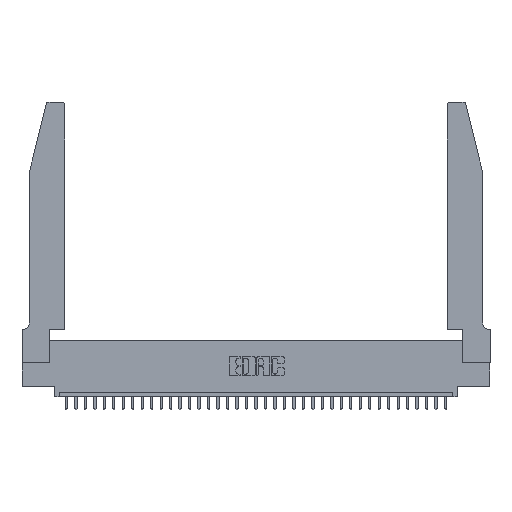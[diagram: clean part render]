
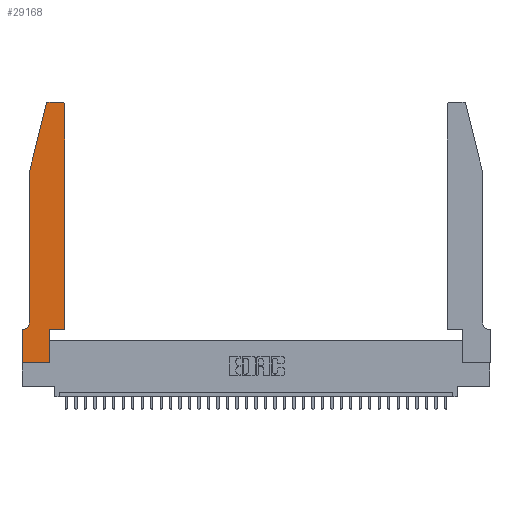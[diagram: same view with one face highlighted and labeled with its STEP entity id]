
A CAD part, top view. The second image highlights one B-rep face of the part: STEP entity #29168.
In plain terms, the highlighted planar face has unit normal (0, 0, 1).
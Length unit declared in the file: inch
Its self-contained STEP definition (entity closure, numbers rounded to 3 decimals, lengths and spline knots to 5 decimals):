
#241 = CARTESIAN_POINT ( 'NONE',  ( 0.0755, 0.42, 0.37 ) ) ;
#341 = EDGE_CURVE ( 'NONE', #12670, #24252, #7398, .T. ) ;
#362 = EDGE_CURVE ( 'NONE', #797, #8042, #8285, .T. ) ;
#366 = DIRECTION ( 'NONE',  ( 0., -1., 0. ) ) ;
#797 = VERTEX_POINT ( 'NONE', #11339 ) ;
#2567 = CARTESIAN_POINT ( 'NONE',  ( 0.2865, 0.35, 0.37 ) ) ;
#3261 = VERTEX_POINT ( 'NONE', #241 ) ;
#4064 = VECTOR ( 'NONE', #11460, 39.37008 ) ;
#4158 = CARTESIAN_POINT ( 'NONE',  ( 0.4505, 0.35, 0.37 ) ) ;
#4185 = ORIENTED_EDGE ( 'NONE', *, *, #7648, .T. ) ;
#4547 = DIRECTION ( 'NONE',  ( -1., 0., 0. ) ) ;
#5834 = LINE ( 'NONE', #22828, #4064 ) ;
#6407 = DIRECTION ( 'NONE',  ( -1., 0., 0. ) ) ;
#6819 = CARTESIAN_POINT ( 'NONE',  ( 0.0755, 2., 0.37 ) ) ;
#6827 = FACE_OUTER_BOUND ( 'NONE', #21174, .T. ) ;
#6879 = DIRECTION ( 'NONE',  ( 1., 0., 0. ) ) ;
#7135 = CARTESIAN_POINT ( 'NONE',  ( 0.4205, 2.72, 0.37 ) ) ;
#7398 = LINE ( 'NONE', #17165, #31655 ) ;
#7491 = DIRECTION ( 'NONE',  ( 0., 0., -1. ) ) ;
#7648 = EDGE_CURVE ( 'NONE', #17571, #33797, #11911, .T. ) ;
#7782 = AXIS2_PLACEMENT_3D ( 'NONE', #21209, #7491, #4547 ) ;
#8014 = VERTEX_POINT ( 'NONE', #6819 ) ;
#8042 = VERTEX_POINT ( 'NONE', #15754 ) ;
#8096 = CARTESIAN_POINT ( 'NONE',  ( 0.0055, 0.35, 0.37 ) ) ;
#8285 = LINE ( 'NONE', #28134, #21728 ) ;
#8612 = DIRECTION ( 'NONE',  ( -0.239, -0.971, 0. ) ) ;
#9207 = LINE ( 'NONE', #25236, #26567 ) ;
#9982 = EDGE_CURVE ( 'NONE', #12471, #8014, #9207, .T. ) ;
#10126 = DIRECTION ( 'NONE',  ( 1., 0., 0. ) ) ;
#10306 = EDGE_CURVE ( 'NONE', #33797, #12670, #18349, .T. ) ;
#10959 = LINE ( 'NONE', #15332, #23095 ) ;
#11264 = ORIENTED_EDGE ( 'NONE', *, *, #26913, .T. ) ;
#11339 = CARTESIAN_POINT ( 'NONE',  ( 0.4205, 2.75, 0.37 ) ) ;
#11460 = DIRECTION ( 'NONE',  ( 1., 0., 0. ) ) ;
#11486 = ORIENTED_EDGE ( 'NONE', *, *, #341, .T. ) ;
#11681 = DIRECTION ( 'NONE',  ( -1., 0., 0. ) ) ;
#11911 = LINE ( 'NONE', #14180, #27510 ) ;
#12445 = VERTEX_POINT ( 'NONE', #26707 ) ;
#12471 = VERTEX_POINT ( 'NONE', #34556 ) ;
#12670 = VERTEX_POINT ( 'NONE', #33101 ) ;
#13048 = EDGE_CURVE ( 'NONE', #12445, #797, #20366, .T. ) ;
#13626 = DIRECTION ( 'NONE',  ( 1., 0., 0. ) ) ;
#14049 = AXIS2_PLACEMENT_3D ( 'NONE', #24625, #27410, #13626 ) ;
#14180 = CARTESIAN_POINT ( 'NONE',  ( 0., 0., 0.37 ) ) ;
#15332 = CARTESIAN_POINT ( 'NONE',  ( 0.0755, 0.35, 0.37 ) ) ;
#15754 = CARTESIAN_POINT ( 'NONE',  ( 0.284, 2.75, 0.37 ) ) ;
#16940 = CARTESIAN_POINT ( 'NONE',  ( 0.0755, 2., 0.37 ) ) ;
#17165 = CARTESIAN_POINT ( 'NONE',  ( 0.2865, 0.35, 0.37 ) ) ;
#17571 = VERTEX_POINT ( 'NONE', #25954 ) ;
#17770 = LINE ( 'NONE', #28290, #35871 ) ;
#18232 = VERTEX_POINT ( 'NONE', #4158 ) ;
#18349 = LINE ( 'NONE', #31943, #21352 ) ;
#18354 = DIRECTION ( 'NONE',  ( 1., 0., 0. ) ) ;
#18426 = ORIENTED_EDGE ( 'NONE', *, *, #30780, .T. ) ;
#19891 = EDGE_CURVE ( 'NONE', #8042, #12471, #26761, .T. ) ;
#20366 = CIRCLE ( 'NONE', #30812, 0.03 ) ;
#20556 = AXIS2_PLACEMENT_3D ( 'NONE', #26854, #29498, #10126 ) ;
#21022 = ORIENTED_EDGE ( 'NONE', *, *, #10306, .T. ) ;
#21174 = EDGE_LOOP ( 'NONE', ( #32458, #24614, #34745, #24854, #18426, #34937, #4185, #21022, #11486, #31013, #11264, #32184 ) ) ;
#21209 = CARTESIAN_POINT ( 'NONE',  ( 0.0055, 0.42, 0.37 ) ) ;
#21352 = VECTOR ( 'NONE', #6879, 39.37008 ) ;
#21728 = VECTOR ( 'NONE', #11681, 39.37008 ) ;
#22462 = VERTEX_POINT ( 'NONE', #8096 ) ;
#22752 = DIRECTION ( 'NONE',  ( 0., -1., 0. ) ) ;
#22828 = CARTESIAN_POINT ( 'NONE',  ( 0.4505, 0.35, 0.37 ) ) ;
#23095 = VECTOR ( 'NONE', #6407, 39.37008 ) ;
#24252 = VERTEX_POINT ( 'NONE', #2567 ) ;
#24614 = ORIENTED_EDGE ( 'NONE', *, *, #19891, .T. ) ;
#24625 = CARTESIAN_POINT ( 'NONE',  ( 0.284, 2.72, 0.37 ) ) ;
#24850 = LINE ( 'NONE', #16940, #30884 ) ;
#24854 = ORIENTED_EDGE ( 'NONE', *, *, #35539, .T. ) ;
#25236 = CARTESIAN_POINT ( 'NONE',  ( 0.0755, 2., 0.37 ) ) ;
#25468 = DIRECTION ( 'NONE',  ( 0., 1., 0. ) ) ;
#25954 = CARTESIAN_POINT ( 'NONE',  ( 0., 0.35, 0.37 ) ) ;
#26567 = VECTOR ( 'NONE', #8612, 39.37008 ) ;
#26707 = CARTESIAN_POINT ( 'NONE',  ( 0.4505, 2.72, 0.37 ) ) ;
#26761 = CIRCLE ( 'NONE', #14049, 0.03 ) ;
#26854 = CARTESIAN_POINT ( 'NONE',  ( 0., 0.35, 0.37 ) ) ;
#26913 = EDGE_CURVE ( 'NONE', #18232, #12445, #17770, .T. ) ;
#27410 = DIRECTION ( 'NONE',  ( 0., 0., 1. ) ) ;
#27510 = VECTOR ( 'NONE', #22752, 39.37008 ) ;
#27727 = CARTESIAN_POINT ( 'NONE',  ( 0., 0., 0.37 ) ) ;
#28134 = CARTESIAN_POINT ( 'NONE',  ( 0.2605, 2.75, 0.37 ) ) ;
#28290 = CARTESIAN_POINT ( 'NONE',  ( 0.4505, 0.35, 0.37 ) ) ;
#29168 = ADVANCED_FACE ( 'NONE', ( #6827 ), #32751, .T. ) ;
#29498 = DIRECTION ( 'NONE',  ( 0., 0., 1. ) ) ;
#30780 = EDGE_CURVE ( 'NONE', #3261, #22462, #34928, .T. ) ;
#30812 = AXIS2_PLACEMENT_3D ( 'NONE', #7135, #34873, #18354 ) ;
#30884 = VECTOR ( 'NONE', #366, 39.37008 ) ;
#31013 = ORIENTED_EDGE ( 'NONE', *, *, #31357, .T. ) ;
#31357 = EDGE_CURVE ( 'NONE', #24252, #18232, #5834, .T. ) ;
#31655 = VECTOR ( 'NONE', #25468, 39.37008 ) ;
#31943 = CARTESIAN_POINT ( 'NONE',  ( 0., 0., 0.37 ) ) ;
#32184 = ORIENTED_EDGE ( 'NONE', *, *, #13048, .T. ) ;
#32458 = ORIENTED_EDGE ( 'NONE', *, *, #362, .T. ) ;
#32751 = PLANE ( 'NONE',  #20556 ) ;
#33101 = CARTESIAN_POINT ( 'NONE',  ( 0.2865, 0., 0.37 ) ) ;
#33614 = DIRECTION ( 'NONE',  ( 0., 1., 0. ) ) ;
#33797 = VERTEX_POINT ( 'NONE', #27727 ) ;
#34556 = CARTESIAN_POINT ( 'NONE',  ( 0.25487, 2.72718, 0.37 ) ) ;
#34745 = ORIENTED_EDGE ( 'NONE', *, *, #9982, .T. ) ;
#34873 = DIRECTION ( 'NONE',  ( 0., 0., 1. ) ) ;
#34928 = CIRCLE ( 'NONE', #7782, 0.07 ) ;
#34937 = ORIENTED_EDGE ( 'NONE', *, *, #35731, .T. ) ;
#35539 = EDGE_CURVE ( 'NONE', #8014, #3261, #24850, .T. ) ;
#35731 = EDGE_CURVE ( 'NONE', #22462, #17571, #10959, .T. ) ;
#35871 = VECTOR ( 'NONE', #33614, 39.37008 ) ;
